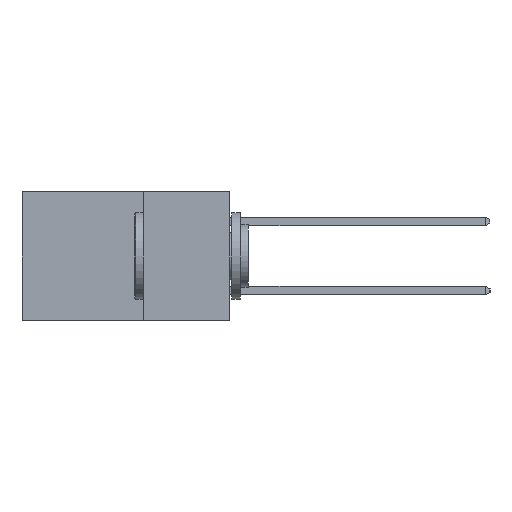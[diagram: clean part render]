
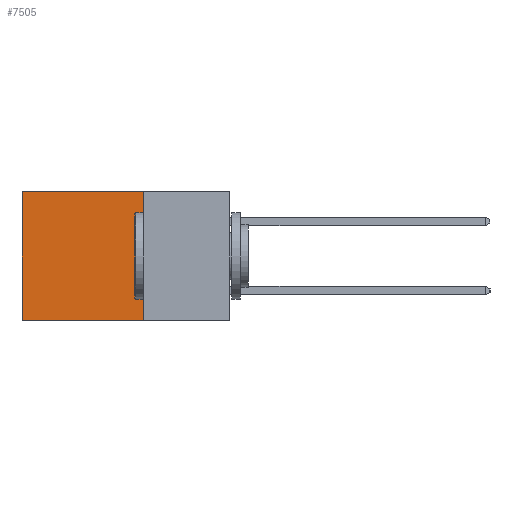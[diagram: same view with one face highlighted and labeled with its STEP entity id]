
A CAD part, left-side view. The second image highlights one B-rep face of the part: STEP entity #7505.
In plain terms, the highlighted planar face has unit normal (-1, 0, 0).
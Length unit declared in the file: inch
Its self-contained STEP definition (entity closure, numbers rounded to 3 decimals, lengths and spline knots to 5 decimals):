
#293 = LINE ( 'NONE', #4088, #13674 ) ;
#550 = EDGE_CURVE ( 'NONE', #8147, #893, #9880, .T. ) ;
#893 = VERTEX_POINT ( 'NONE', #2883 ) ;
#1095 = AXIS2_PLACEMENT_3D ( 'NONE', #13635, #6020, #14932 ) ;
#2195 = LINE ( 'NONE', #8880, #12457 ) ;
#2883 = CARTESIAN_POINT ( 'NONE',  ( 0.2615, 0.6, 0. ) ) ;
#3276 = ORIENTED_EDGE ( 'NONE', *, *, #550, .T. ) ;
#3592 = CARTESIAN_POINT ( 'NONE',  ( 0.2615, 0.25, -0.37 ) ) ;
#4088 = CARTESIAN_POINT ( 'NONE',  ( 0.2615, 0.25, -0.37 ) ) ;
#4489 = CARTESIAN_POINT ( 'NONE',  ( 0.2615, 0.6, -0.37 ) ) ;
#4514 = VERTEX_POINT ( 'NONE', #8752 ) ;
#4897 = ORIENTED_EDGE ( 'NONE', *, *, #6974, .T. ) ;
#5961 = PLANE ( 'NONE',  #1095 ) ;
#6020 = DIRECTION ( 'NONE',  ( 1., 0., 0. ) ) ;
#6974 = EDGE_CURVE ( 'NONE', #893, #14930, #2195, .T. ) ;
#7505 = ADVANCED_FACE ( 'NONE', ( #14215 ), #5961, .F. ) ;
#8147 = VERTEX_POINT ( 'NONE', #13500 ) ;
#8752 = CARTESIAN_POINT ( 'NONE',  ( 0.2615, 0.25, -0.37 ) ) ;
#8880 = CARTESIAN_POINT ( 'NONE',  ( 0.2615, 0.6, -0.37 ) ) ;
#9880 = LINE ( 'NONE', #10481, #12473 ) ;
#10127 = VECTOR ( 'NONE', #11256, 39.37008 ) ;
#10481 = CARTESIAN_POINT ( 'NONE',  ( 0.2615, 0.25, 0. ) ) ;
#10696 = ORIENTED_EDGE ( 'NONE', *, *, #16013, .F. ) ;
#11256 = DIRECTION ( 'NONE',  ( 0., 0., -1. ) ) ;
#11747 = DIRECTION ( 'NONE',  ( 0., 1., 0. ) ) ;
#12263 = EDGE_CURVE ( 'NONE', #4514, #14930, #293, .T. ) ;
#12457 = VECTOR ( 'NONE', #16486, 39.37008 ) ;
#12473 = VECTOR ( 'NONE', #13044, 39.37008 ) ;
#13044 = DIRECTION ( 'NONE',  ( 0., 1., 0. ) ) ;
#13500 = CARTESIAN_POINT ( 'NONE',  ( 0.2615, 0.25, 0. ) ) ;
#13504 = LINE ( 'NONE', #3592, #10127 ) ;
#13635 = CARTESIAN_POINT ( 'NONE',  ( 0.2615, 0.25, -0.37 ) ) ;
#13674 = VECTOR ( 'NONE', #11747, 39.37008 ) ;
#14057 = EDGE_LOOP ( 'NONE', ( #4897, #14840, #10696, #3276 ) ) ;
#14215 = FACE_OUTER_BOUND ( 'NONE', #14057, .T. ) ;
#14840 = ORIENTED_EDGE ( 'NONE', *, *, #12263, .F. ) ;
#14930 = VERTEX_POINT ( 'NONE', #4489 ) ;
#14932 = DIRECTION ( 'NONE',  ( 0., 0., -1. ) ) ;
#16013 = EDGE_CURVE ( 'NONE', #8147, #4514, #13504, .T. ) ;
#16486 = DIRECTION ( 'NONE',  ( 0., 0., -1. ) ) ;
